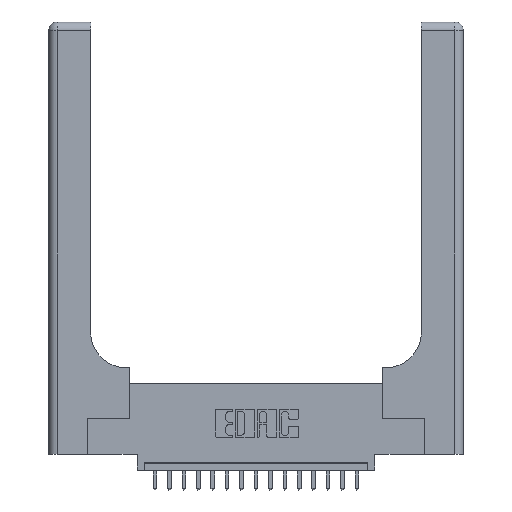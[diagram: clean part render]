
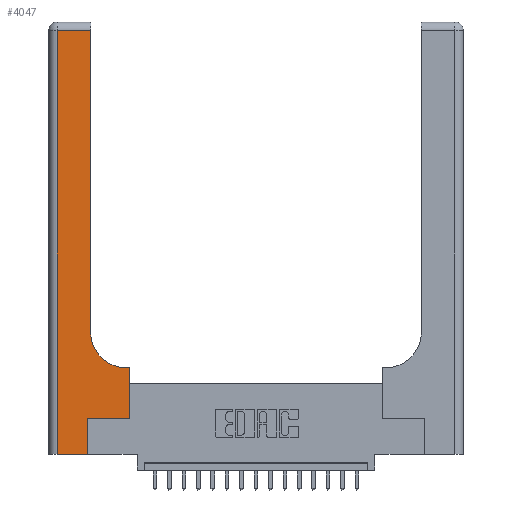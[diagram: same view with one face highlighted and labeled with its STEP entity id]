
A CAD part, top view. The second image highlights one B-rep face of the part: STEP entity #4047.
In plain terms, the highlighted planar face has unit normal (0, 0, 1).
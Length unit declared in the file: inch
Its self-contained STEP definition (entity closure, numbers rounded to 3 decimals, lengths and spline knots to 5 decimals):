
#342 = LINE ( 'NONE', #4153, #17476 ) ;
#1394 = CARTESIAN_POINT ( 'NONE',  ( 0.269, 0.25, 0.37 ) ) ;
#1502 = PLANE ( 'NONE',  #12345 ) ;
#2029 = VECTOR ( 'NONE', #8619, 39.37008 ) ;
#2132 = ORIENTED_EDGE ( 'NONE', *, *, #2389, .T. ) ;
#2369 = VECTOR ( 'NONE', #10284, 39.37008 ) ;
#2389 = EDGE_CURVE ( 'NONE', #3738, #9925, #6444, .T. ) ;
#2690 = ORIENTED_EDGE ( 'NONE', *, *, #13852, .T. ) ;
#2723 = CARTESIAN_POINT ( 'NONE',  ( 0.5585, 0.25, 0.37 ) ) ;
#2747 = VECTOR ( 'NONE', #18968, 39.37008 ) ;
#2795 = ORIENTED_EDGE ( 'NONE', *, *, #17205, .T. ) ;
#3229 = CARTESIAN_POINT ( 'NONE',  ( 0.5415, 0.85, 0.37 ) ) ;
#3738 = VERTEX_POINT ( 'NONE', #19771 ) ;
#4033 = CARTESIAN_POINT ( 'NONE',  ( 0.2915, 2.94, 0.37 ) ) ;
#4047 = ADVANCED_FACE ( 'NONE', ( #8056 ), #1502, .F. ) ;
#4153 = CARTESIAN_POINT ( 'NONE',  ( 0.269, 0., 0.37 ) ) ;
#4757 = CARTESIAN_POINT ( 'NONE',  ( 0.5585, 0.6, 0.37 ) ) ;
#4809 = ORIENTED_EDGE ( 'NONE', *, *, #5182, .T. ) ;
#5105 = VECTOR ( 'NONE', #5254, 39.37008 ) ;
#5128 = VERTEX_POINT ( 'NONE', #4757 ) ;
#5182 = EDGE_CURVE ( 'NONE', #10396, #10694, #9496, .T. ) ;
#5254 = DIRECTION ( 'NONE',  ( 0., -1., 0. ) ) ;
#6381 = CARTESIAN_POINT ( 'NONE',  ( 0.269, 0., 0.37 ) ) ;
#6444 = LINE ( 'NONE', #14106, #2747 ) ;
#6490 = EDGE_CURVE ( 'NONE', #9925, #10396, #342, .T. ) ;
#6700 = LINE ( 'NONE', #14749, #2029 ) ;
#7448 = EDGE_CURVE ( 'NONE', #5128, #18200, #6700, .T. ) ;
#7789 = VECTOR ( 'NONE', #10671, 39.37008 ) ;
#8022 = DIRECTION ( 'NONE',  ( 1., 0., 0. ) ) ;
#8056 = FACE_OUTER_BOUND ( 'NONE', #17984, .T. ) ;
#8451 = DIRECTION ( 'NONE',  ( 1., 0., 0. ) ) ;
#8619 = DIRECTION ( 'NONE',  ( -1., 0., 0. ) ) ;
#8670 = ORIENTED_EDGE ( 'NONE', *, *, #18452, .T. ) ;
#9021 = VECTOR ( 'NONE', #13598, 39.37008 ) ;
#9496 = LINE ( 'NONE', #14464, #16067 ) ;
#9925 = VERTEX_POINT ( 'NONE', #6381 ) ;
#10036 = CARTESIAN_POINT ( 'NONE',  ( 0.5585, 0.25, 0.37 ) ) ;
#10284 = DIRECTION ( 'NONE',  ( 0., 1., 0. ) ) ;
#10396 = VERTEX_POINT ( 'NONE', #1394 ) ;
#10671 = DIRECTION ( 'NONE',  ( -1., 0., 0. ) ) ;
#10694 = VERTEX_POINT ( 'NONE', #10036 ) ;
#10721 = VERTEX_POINT ( 'NONE', #17890 ) ;
#10960 = DIRECTION ( 'NONE',  ( -1., 0., 0. ) ) ;
#11181 = LINE ( 'NONE', #18059, #2369 ) ;
#11679 = LINE ( 'NONE', #2723, #9021 ) ;
#11837 = ORIENTED_EDGE ( 'NONE', *, *, #6490, .T. ) ;
#12086 = AXIS2_PLACEMENT_3D ( 'NONE', #3229, #14170, #8022 ) ;
#12276 = CARTESIAN_POINT ( 'NONE',  ( 0.5415, 0.6, 0.37 ) ) ;
#12345 = AXIS2_PLACEMENT_3D ( 'NONE', #12452, #14026, #10960 ) ;
#12393 = ORIENTED_EDGE ( 'NONE', *, *, #13533, .T. ) ;
#12452 = CARTESIAN_POINT ( 'NONE',  ( 0., 3., 0.37 ) ) ;
#13533 = EDGE_CURVE ( 'NONE', #18200, #10721, #17567, .T. ) ;
#13598 = DIRECTION ( 'NONE',  ( 0., 1., 0. ) ) ;
#13852 = EDGE_CURVE ( 'NONE', #16827, #16835, #20263, .T. ) ;
#14026 = DIRECTION ( 'NONE',  ( 0., 0., -1. ) ) ;
#14106 = CARTESIAN_POINT ( 'NONE',  ( 0., 0., 0.37 ) ) ;
#14170 = DIRECTION ( 'NONE',  ( 0., 0., -1. ) ) ;
#14464 = CARTESIAN_POINT ( 'NONE',  ( 0.269, 0.25, 0.37 ) ) ;
#14513 = ORIENTED_EDGE ( 'NONE', *, *, #7448, .T. ) ;
#14749 = CARTESIAN_POINT ( 'NONE',  ( 0.2915, 0.6, 0.37 ) ) ;
#15736 = CARTESIAN_POINT ( 'NONE',  ( 0.06, 3., 0.37 ) ) ;
#16067 = VECTOR ( 'NONE', #8451, 39.37008 ) ;
#16827 = VERTEX_POINT ( 'NONE', #4033 ) ;
#16835 = VERTEX_POINT ( 'NONE', #18138 ) ;
#17205 = EDGE_CURVE ( 'NONE', #16835, #3738, #19054, .T. ) ;
#17476 = VECTOR ( 'NONE', #18304, 39.37008 ) ;
#17484 = ORIENTED_EDGE ( 'NONE', *, *, #17528, .T. ) ;
#17528 = EDGE_CURVE ( 'NONE', #10694, #5128, #11679, .T. ) ;
#17567 = CIRCLE ( 'NONE', #12086, 0.25 ) ;
#17890 = CARTESIAN_POINT ( 'NONE',  ( 0.2915, 0.85, 0.37 ) ) ;
#17984 = EDGE_LOOP ( 'NONE', ( #8670, #2690, #2795, #2132, #11837, #4809, #17484, #14513, #12393 ) ) ;
#18059 = CARTESIAN_POINT ( 'NONE',  ( 0.2915, 3., 0.37 ) ) ;
#18138 = CARTESIAN_POINT ( 'NONE',  ( 0.06, 2.94, 0.37 ) ) ;
#18200 = VERTEX_POINT ( 'NONE', #12276 ) ;
#18304 = DIRECTION ( 'NONE',  ( 0., 1., 0. ) ) ;
#18452 = EDGE_CURVE ( 'NONE', #10721, #16827, #11181, .T. ) ;
#18968 = DIRECTION ( 'NONE',  ( 1., 0., 0. ) ) ;
#19054 = LINE ( 'NONE', #15736, #5105 ) ;
#19771 = CARTESIAN_POINT ( 'NONE',  ( 0.06, 0., 0.37 ) ) ;
#19892 = CARTESIAN_POINT ( 'NONE',  ( 0., 2.94, 0.37 ) ) ;
#20263 = LINE ( 'NONE', #19892, #7789 ) ;
